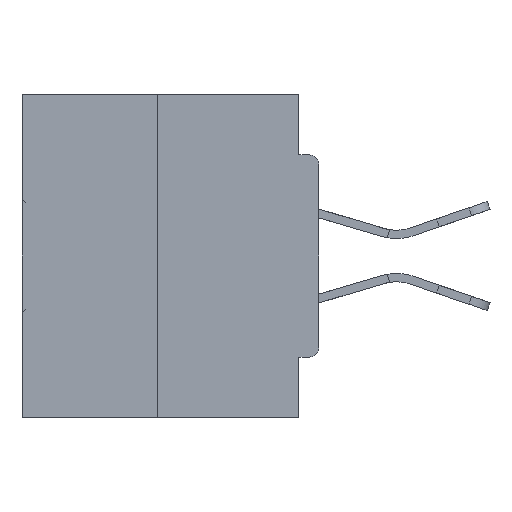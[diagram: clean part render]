
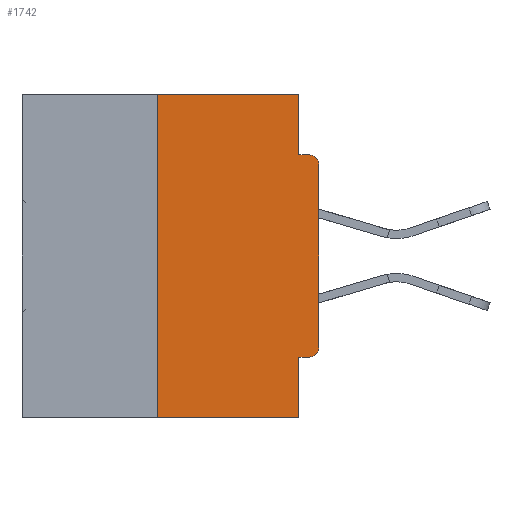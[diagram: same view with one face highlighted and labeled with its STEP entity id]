
A CAD part, left-side view. The second image highlights one B-rep face of the part: STEP entity #1742.
In plain terms, the highlighted planar face has unit normal (-1, 0, 0).
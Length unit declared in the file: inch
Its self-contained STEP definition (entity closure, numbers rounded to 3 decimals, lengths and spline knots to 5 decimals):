
#107 = LINE ( 'NONE', #15748, #29652 ) ;
#1593 = VECTOR ( 'NONE', #38786, 39.37008 ) ;
#1673 = VERTEX_POINT ( 'NONE', #29869 ) ;
#1742 = ADVANCED_FACE ( 'NONE', ( #43967 ), #5010, .F. ) ;
#2306 = DIRECTION ( 'NONE',  ( 0., 0., -1. ) ) ;
#2329 = EDGE_CURVE ( 'NONE', #11530, #10980, #24585, .T. ) ;
#2844 = VERTEX_POINT ( 'NONE', #32129 ) ;
#3188 = CARTESIAN_POINT ( 'NONE',  ( 0., 0.25, 0. ) ) ;
#4370 = LINE ( 'NONE', #36389, #36180 ) ;
#5010 = PLANE ( 'NONE',  #42126 ) ;
#5735 = CARTESIAN_POINT ( 'NONE',  ( 0., 0.25, -0.5 ) ) ;
#6489 = LINE ( 'NONE', #37370, #38825 ) ;
#6602 = EDGE_CURVE ( 'NONE', #34174, #13106, #6489, .T. ) ;
#7163 = EDGE_CURVE ( 'NONE', #34174, #1673, #34740, .T. ) ;
#7915 = VECTOR ( 'NONE', #27857, 39.37008 ) ;
#8869 = CARTESIAN_POINT ( 'NONE',  ( 0., 0., -0.3915 ) ) ;
#8976 = CARTESIAN_POINT ( 'NONE',  ( 0., 0.031, -0.0935 ) ) ;
#9364 = EDGE_CURVE ( 'NONE', #11945, #2844, #14551, .T. ) ;
#9935 = CARTESIAN_POINT ( 'NONE',  ( 0., 0.015, -0.1085 ) ) ;
#10037 = EDGE_CURVE ( 'NONE', #1673, #20078, #4370, .T. ) ;
#10085 = DIRECTION ( 'NONE',  ( 0., 0., -1. ) ) ;
#10660 = LINE ( 'NONE', #24702, #1593 ) ;
#10980 = VERTEX_POINT ( 'NONE', #8869 ) ;
#11134 = VERTEX_POINT ( 'NONE', #13428 ) ;
#11259 = DIRECTION ( 'NONE',  ( 0., -1., 0. ) ) ;
#11530 = VERTEX_POINT ( 'NONE', #16377 ) ;
#11945 = VERTEX_POINT ( 'NONE', #8976 ) ;
#12430 = ORIENTED_EDGE ( 'NONE', *, *, #34008, .F. ) ;
#13106 = VERTEX_POINT ( 'NONE', #33335 ) ;
#13270 = ORIENTED_EDGE ( 'NONE', *, *, #7163, .F. ) ;
#13428 = CARTESIAN_POINT ( 'NONE',  ( 0., 0.031, -0.4065 ) ) ;
#14228 = DIRECTION ( 'NONE',  ( -1., 0., 0. ) ) ;
#14551 = LINE ( 'NONE', #38535, #24356 ) ;
#14664 = ORIENTED_EDGE ( 'NONE', *, *, #9364, .F. ) ;
#14803 = ORIENTED_EDGE ( 'NONE', *, *, #10037, .F. ) ;
#15060 = DIRECTION ( 'NONE',  ( 0., 1., 0. ) ) ;
#15138 = VECTOR ( 'NONE', #42830, 39.37008 ) ;
#15748 = CARTESIAN_POINT ( 'NONE',  ( 0., 0., -0.4065 ) ) ;
#16377 = CARTESIAN_POINT ( 'NONE',  ( 0., 0.015, -0.4065 ) ) ;
#17046 = DIRECTION ( 'NONE',  ( 0., 0., -1. ) ) ;
#17391 = ORIENTED_EDGE ( 'NONE', *, *, #6602, .T. ) ;
#18562 = LINE ( 'NONE', #25036, #15138 ) ;
#19753 = CARTESIAN_POINT ( 'NONE',  ( 0., 0.031, 0. ) ) ;
#20078 = VERTEX_POINT ( 'NONE', #38236 ) ;
#20295 = AXIS2_PLACEMENT_3D ( 'NONE', #9935, #14228, #17046 ) ;
#20719 = DIRECTION ( 'NONE',  ( 0., -1., 0. ) ) ;
#22178 = EDGE_CURVE ( 'NONE', #10980, #43897, #18562, .T. ) ;
#22865 = ORIENTED_EDGE ( 'NONE', *, *, #2329, .T. ) ;
#23166 = DIRECTION ( 'NONE',  ( 1., 0., 0. ) ) ;
#24356 = VECTOR ( 'NONE', #24683, 39.37008 ) ;
#24585 = CIRCLE ( 'NONE', #34896, 0.015 ) ;
#24683 = DIRECTION ( 'NONE',  ( 0., -1., 0. ) ) ;
#24702 = CARTESIAN_POINT ( 'NONE',  ( 0., 0.031, -0.5 ) ) ;
#25036 = CARTESIAN_POINT ( 'NONE',  ( 0., 0., 0. ) ) ;
#25725 = EDGE_CURVE ( 'NONE', #43897, #2844, #35034, .T. ) ;
#26418 = CARTESIAN_POINT ( 'NONE',  ( 0., 0.46, 0. ) ) ;
#27202 = DIRECTION ( 'NONE',  ( -1., 0., 0. ) ) ;
#27563 = CARTESIAN_POINT ( 'NONE',  ( 0., 0., -0.1085 ) ) ;
#27857 = DIRECTION ( 'NONE',  ( 0., 0., 1. ) ) ;
#29652 = VECTOR ( 'NONE', #15060, 39.37008 ) ;
#29869 = CARTESIAN_POINT ( 'NONE',  ( 0., 0.25, 0. ) ) ;
#31130 = ORIENTED_EDGE ( 'NONE', *, *, #25725, .T. ) ;
#32129 = CARTESIAN_POINT ( 'NONE',  ( 0., 0.015, -0.0935 ) ) ;
#33335 = CARTESIAN_POINT ( 'NONE',  ( 0., 0.031, -0.5 ) ) ;
#33550 = DIRECTION ( 'NONE',  ( 0., 0., -1. ) ) ;
#34008 = EDGE_CURVE ( 'NONE', #20078, #11945, #40762, .T. ) ;
#34174 = VERTEX_POINT ( 'NONE', #5735 ) ;
#34740 = LINE ( 'NONE', #3188, #7915 ) ;
#34896 = AXIS2_PLACEMENT_3D ( 'NONE', #40835, #27202, #2306 ) ;
#35034 = CIRCLE ( 'NONE', #20295, 0.015 ) ;
#35956 = EDGE_CURVE ( 'NONE', #11530, #11134, #107, .T. ) ;
#36118 = ORIENTED_EDGE ( 'NONE', *, *, #22178, .T. ) ;
#36180 = VECTOR ( 'NONE', #11259, 39.37008 ) ;
#36389 = CARTESIAN_POINT ( 'NONE',  ( 0., 0.46, 0. ) ) ;
#37370 = CARTESIAN_POINT ( 'NONE',  ( 0., 0.46, -0.5 ) ) ;
#37620 = VECTOR ( 'NONE', #10085, 39.37008 ) ;
#38236 = CARTESIAN_POINT ( 'NONE',  ( 0., 0.031, 0. ) ) ;
#38535 = CARTESIAN_POINT ( 'NONE',  ( 0., 0., -0.0935 ) ) ;
#38786 = DIRECTION ( 'NONE',  ( 0., 0., -1. ) ) ;
#38825 = VECTOR ( 'NONE', #20719, 39.37008 ) ;
#39314 = EDGE_CURVE ( 'NONE', #11134, #13106, #10660, .T. ) ;
#40762 = LINE ( 'NONE', #19753, #37620 ) ;
#40835 = CARTESIAN_POINT ( 'NONE',  ( 0., 0.015, -0.3915 ) ) ;
#41735 = ORIENTED_EDGE ( 'NONE', *, *, #39314, .F. ) ;
#42126 = AXIS2_PLACEMENT_3D ( 'NONE', #26418, #23166, #33550 ) ;
#42830 = DIRECTION ( 'NONE',  ( 0., 0., 1. ) ) ;
#43897 = VERTEX_POINT ( 'NONE', #27563 ) ;
#43967 = FACE_OUTER_BOUND ( 'NONE', #45133, .T. ) ;
#44669 = ORIENTED_EDGE ( 'NONE', *, *, #35956, .F. ) ;
#45133 = EDGE_LOOP ( 'NONE', ( #14803, #13270, #17391, #41735, #44669, #22865, #36118, #31130, #14664, #12430 ) ) ;
